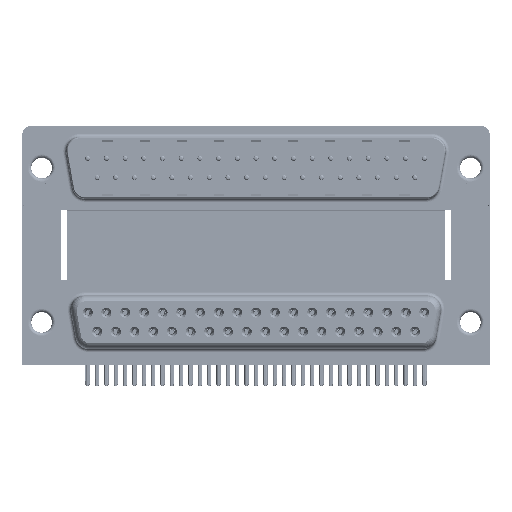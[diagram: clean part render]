
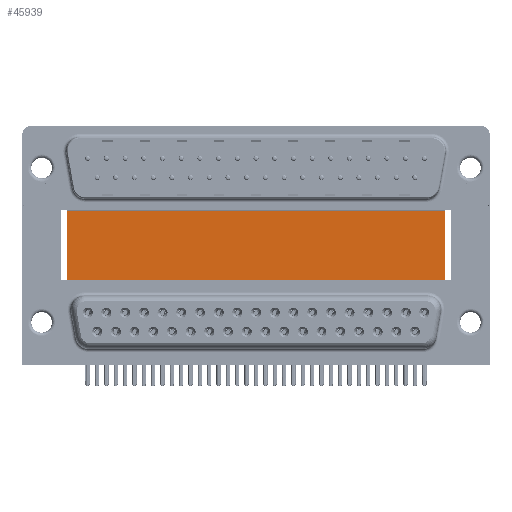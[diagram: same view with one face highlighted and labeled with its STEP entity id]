
A CAD part, top view. The second image highlights one B-rep face of the part: STEP entity #45939.
In plain terms, the highlighted planar face has unit normal (0, 0, 1).
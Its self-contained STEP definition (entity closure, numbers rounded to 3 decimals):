
#4344 = LINE ( 'NONE', #51612, #32987 ) ;
#5172 = LINE ( 'NONE', #47321, #12176 ) ;
#5629 = ORIENTED_EDGE ( 'NONE', *, *, #32291, .T. ) ;
#5788 = EDGE_LOOP ( 'NONE', ( #31692, #24838, #38463, #5629 ) ) ;
#9979 = DIRECTION ( 'NONE',  ( 0., -1., 0. ) ) ;
#11769 = VERTEX_POINT ( 'NONE', #44656 ) ;
#12176 = VECTOR ( 'NONE', #9979, 1000. ) ;
#22632 = PLANE ( 'NONE',  #57093 ) ;
#24838 = ORIENTED_EDGE ( 'NONE', *, *, #47161, .F. ) ;
#31692 = ORIENTED_EDGE ( 'NONE', *, *, #66273, .T. ) ;
#32227 = CARTESIAN_POINT ( 'NONE',  ( 3.79, 16.585, -12. ) ) ;
#32291 = EDGE_CURVE ( 'NONE', #42133, #11769, #42284, .T. ) ;
#32646 = EDGE_CURVE ( 'NONE', #42133, #65234, #36077, .T. ) ;
#32987 = VECTOR ( 'NONE', #46492, 1000. ) ;
#33007 = DIRECTION ( 'NONE',  ( 0., -1., 0. ) ) ;
#33340 = CARTESIAN_POINT ( 'NONE',  ( 59.71, 16.585, -12. ) ) ;
#36077 = LINE ( 'NONE', #51810, #41753 ) ;
#37501 = CARTESIAN_POINT ( 'NONE',  ( 3.79, 16.585, -12. ) ) ;
#38463 = ORIENTED_EDGE ( 'NONE', *, *, #32646, .F. ) ;
#41753 = VECTOR ( 'NONE', #62402, 1000. ) ;
#42133 = VERTEX_POINT ( 'NONE', #59391 ) ;
#42284 = LINE ( 'NONE', #37501, #49425 ) ;
#44368 = VERTEX_POINT ( 'NONE', #66912 ) ;
#44656 = CARTESIAN_POINT ( 'NONE',  ( 3.79, -3.735, -12. ) ) ;
#45939 = ADVANCED_FACE ( 'NONE', ( #47981 ), #22632, .F. ) ;
#46492 = DIRECTION ( 'NONE',  ( 1., 0., 0. ) ) ;
#47161 = EDGE_CURVE ( 'NONE', #65234, #44368, #5172, .T. ) ;
#47321 = CARTESIAN_POINT ( 'NONE',  ( 59.71, 16.585, -12. ) ) ;
#47981 = FACE_OUTER_BOUND ( 'NONE', #5788, .T. ) ;
#49425 = VECTOR ( 'NONE', #33007, 1000. ) ;
#51612 = CARTESIAN_POINT ( 'NONE',  ( 3.79, -3.735, -12. ) ) ;
#51810 = CARTESIAN_POINT ( 'NONE',  ( 3.79, 16.585, -12. ) ) ;
#57093 = AXIS2_PLACEMENT_3D ( 'NONE', #32227, #64389, #57913 ) ;
#57913 = DIRECTION ( 'NONE',  ( -1., 0., 0. ) ) ;
#59391 = CARTESIAN_POINT ( 'NONE',  ( 3.79, 16.585, -12. ) ) ;
#62402 = DIRECTION ( 'NONE',  ( 1., 0., 0. ) ) ;
#64389 = DIRECTION ( 'NONE',  ( 0., 0., -1. ) ) ;
#65234 = VERTEX_POINT ( 'NONE', #33340 ) ;
#66273 = EDGE_CURVE ( 'NONE', #11769, #44368, #4344, .T. ) ;
#66912 = CARTESIAN_POINT ( 'NONE',  ( 59.71, -3.735, -12. ) ) ;
